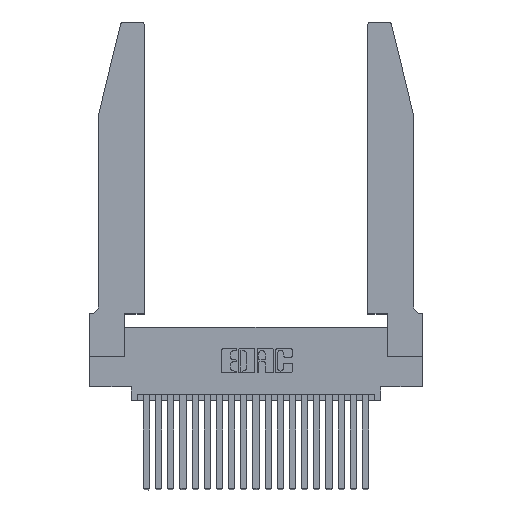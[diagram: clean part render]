
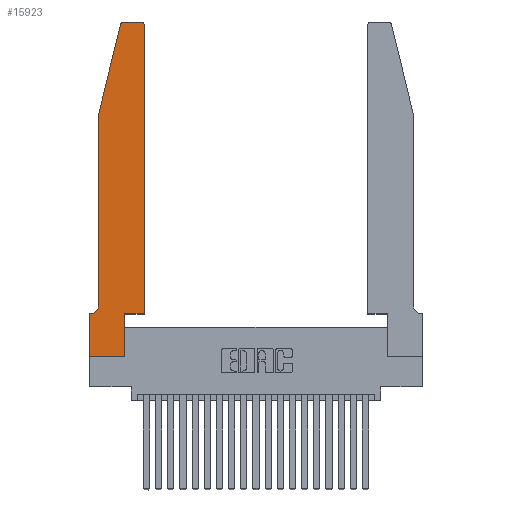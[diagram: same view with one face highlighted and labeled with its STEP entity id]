
A CAD part, top view. The second image highlights one B-rep face of the part: STEP entity #15923.
In plain terms, the highlighted planar face has unit normal (0, 0, 1).
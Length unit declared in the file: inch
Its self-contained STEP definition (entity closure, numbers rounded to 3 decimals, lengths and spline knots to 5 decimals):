
#23 = DIRECTION ( 'NONE',  ( 1., 0., 0. ) ) ;
#68 = EDGE_LOOP ( 'NONE', ( #13215, #6285, #16899, #22281, #315, #334, #8692, #9339, #8426, #6240, #14320, #22237 ) ) ;
#199 = DIRECTION ( 'NONE',  ( 1., 0., 0. ) ) ;
#242 = VECTOR ( 'NONE', #10638, 39.37008 ) ;
#315 = ORIENTED_EDGE ( 'NONE', *, *, #13425, .T. ) ;
#334 = ORIENTED_EDGE ( 'NONE', *, *, #4951, .T. ) ;
#385 = VERTEX_POINT ( 'NONE', #7137 ) ;
#736 = CARTESIAN_POINT ( 'NONE',  ( 0.4505, 0.35, 0.37 ) ) ;
#1230 = VECTOR ( 'NONE', #23, 39.37008 ) ;
#1583 = CARTESIAN_POINT ( 'NONE',  ( 0.4505, 0.35, 0.37 ) ) ;
#1658 = DIRECTION ( 'NONE',  ( 0., 0., 1. ) ) ;
#1879 = VERTEX_POINT ( 'NONE', #16109 ) ;
#2023 = CARTESIAN_POINT ( 'NONE',  ( 0., 0., 0.37 ) ) ;
#2698 = CARTESIAN_POINT ( 'NONE',  ( 0.0755, 2., 0.37 ) ) ;
#2812 = CARTESIAN_POINT ( 'NONE',  ( 0.284, 2.75, 0.37 ) ) ;
#2845 = EDGE_CURVE ( 'NONE', #11661, #4083, #5709, .T. ) ;
#2954 = PLANE ( 'NONE',  #10934 ) ;
#3644 = VECTOR ( 'NONE', #199, 39.37008 ) ;
#3740 = CARTESIAN_POINT ( 'NONE',  ( 0., 0., 0.37 ) ) ;
#3824 = CARTESIAN_POINT ( 'NONE',  ( 0.0755, 2., 0.37 ) ) ;
#4083 = VERTEX_POINT ( 'NONE', #2812 ) ;
#4455 = LINE ( 'NONE', #3824, #17082 ) ;
#4795 = VERTEX_POINT ( 'NONE', #22467 ) ;
#4796 = AXIS2_PLACEMENT_3D ( 'NONE', #5248, #1658, #10400 ) ;
#4951 = EDGE_CURVE ( 'NONE', #19156, #15522, #16598, .T. ) ;
#5170 = CARTESIAN_POINT ( 'NONE',  ( 0.0055, 0.35, 0.37 ) ) ;
#5248 = CARTESIAN_POINT ( 'NONE',  ( 0.284, 2.72, 0.37 ) ) ;
#5652 = EDGE_CURVE ( 'NONE', #4795, #11661, #22323, .T. ) ;
#5709 = LINE ( 'NONE', #21184, #242 ) ;
#5722 = CARTESIAN_POINT ( 'NONE',  ( 0.4505, 0.35, 0.37 ) ) ;
#6138 = DIRECTION ( 'NONE',  ( 1., 0., 0. ) ) ;
#6240 = ORIENTED_EDGE ( 'NONE', *, *, #19174, .T. ) ;
#6285 = ORIENTED_EDGE ( 'NONE', *, *, #20259, .T. ) ;
#6374 = EDGE_CURVE ( 'NONE', #9184, #7392, #6906, .T. ) ;
#6789 = DIRECTION ( 'NONE',  ( -1., 0., 0. ) ) ;
#6906 = LINE ( 'NONE', #3740, #3644 ) ;
#7137 = CARTESIAN_POINT ( 'NONE',  ( 0.25487, 2.72718, 0.37 ) ) ;
#7377 = CARTESIAN_POINT ( 'NONE',  ( 0.2865, 0., 0.37 ) ) ;
#7392 = VERTEX_POINT ( 'NONE', #7377 ) ;
#8208 = CARTESIAN_POINT ( 'NONE',  ( 0., 0.35, 0.37 ) ) ;
#8245 = LINE ( 'NONE', #14918, #15685 ) ;
#8426 = ORIENTED_EDGE ( 'NONE', *, *, #13246, .T. ) ;
#8542 = VERTEX_POINT ( 'NONE', #9794 ) ;
#8692 = ORIENTED_EDGE ( 'NONE', *, *, #11339, .T. ) ;
#9184 = VERTEX_POINT ( 'NONE', #2023 ) ;
#9339 = ORIENTED_EDGE ( 'NONE', *, *, #6374, .T. ) ;
#9432 = EDGE_CURVE ( 'NONE', #19937, #4795, #21313, .T. ) ;
#9520 = DIRECTION ( 'NONE',  ( 0., -1., 0. ) ) ;
#9662 = CIRCLE ( 'NONE', #12365, 0.07 ) ;
#9794 = CARTESIAN_POINT ( 'NONE',  ( 0.0755, 0.42, 0.37 ) ) ;
#10164 = DIRECTION ( 'NONE',  ( 0., 0., 1. ) ) ;
#10400 = DIRECTION ( 'NONE',  ( 1., 0., 0. ) ) ;
#10491 = CARTESIAN_POINT ( 'NONE',  ( 0.4205, 2.75, 0.37 ) ) ;
#10638 = DIRECTION ( 'NONE',  ( -1., 0., 0. ) ) ;
#10934 = AXIS2_PLACEMENT_3D ( 'NONE', #13537, #10164, #22427 ) ;
#11192 = CARTESIAN_POINT ( 'NONE',  ( 0.0055, 0.42, 0.37 ) ) ;
#11339 = EDGE_CURVE ( 'NONE', #15522, #9184, #11368, .T. ) ;
#11368 = LINE ( 'NONE', #14707, #22587 ) ;
#11377 = CARTESIAN_POINT ( 'NONE',  ( 0.4205, 2.72, 0.37 ) ) ;
#11661 = VERTEX_POINT ( 'NONE', #10491 ) ;
#11681 = DIRECTION ( 'NONE',  ( 0., -1., 0. ) ) ;
#11734 = VECTOR ( 'NONE', #11681, 39.37008 ) ;
#11840 = EDGE_CURVE ( 'NONE', #385, #15113, #4455, .T. ) ;
#11990 = VECTOR ( 'NONE', #14680, 39.37008 ) ;
#12365 = AXIS2_PLACEMENT_3D ( 'NONE', #11192, #14843, #21897 ) ;
#12826 = LINE ( 'NONE', #2698, #11734 ) ;
#13215 = ORIENTED_EDGE ( 'NONE', *, *, #2845, .T. ) ;
#13246 = EDGE_CURVE ( 'NONE', #7392, #1879, #8245, .T. ) ;
#13425 = EDGE_CURVE ( 'NONE', #8542, #19156, #9662, .T. ) ;
#13537 = CARTESIAN_POINT ( 'NONE',  ( 0., 0.35, 0.37 ) ) ;
#14320 = ORIENTED_EDGE ( 'NONE', *, *, #9432, .T. ) ;
#14680 = DIRECTION ( 'NONE',  ( 0., 1., 0. ) ) ;
#14707 = CARTESIAN_POINT ( 'NONE',  ( 0., 0., 0.37 ) ) ;
#14843 = DIRECTION ( 'NONE',  ( 0., 0., -1. ) ) ;
#14870 = DIRECTION ( 'NONE',  ( 0., 0., 1. ) ) ;
#14918 = CARTESIAN_POINT ( 'NONE',  ( 0.2865, 0.35, 0.37 ) ) ;
#15113 = VERTEX_POINT ( 'NONE', #21709 ) ;
#15132 = AXIS2_PLACEMENT_3D ( 'NONE', #11377, #14870, #6138 ) ;
#15522 = VERTEX_POINT ( 'NONE', #8208 ) ;
#15685 = VECTOR ( 'NONE', #20204, 39.37008 ) ;
#15923 = ADVANCED_FACE ( 'NONE', ( #18914 ), #2954, .T. ) ;
#16109 = CARTESIAN_POINT ( 'NONE',  ( 0.2865, 0.35, 0.37 ) ) ;
#16598 = LINE ( 'NONE', #17532, #22370 ) ;
#16899 = ORIENTED_EDGE ( 'NONE', *, *, #11840, .T. ) ;
#17082 = VECTOR ( 'NONE', #17824, 39.37008 ) ;
#17532 = CARTESIAN_POINT ( 'NONE',  ( 0.0755, 0.35, 0.37 ) ) ;
#17824 = DIRECTION ( 'NONE',  ( -0.239, -0.971, 0. ) ) ;
#17965 = EDGE_CURVE ( 'NONE', #15113, #8542, #12826, .T. ) ;
#18730 = CIRCLE ( 'NONE', #4796, 0.03 ) ;
#18914 = FACE_OUTER_BOUND ( 'NONE', #68, .T. ) ;
#19156 = VERTEX_POINT ( 'NONE', #5170 ) ;
#19174 = EDGE_CURVE ( 'NONE', #1879, #19937, #21534, .T. ) ;
#19937 = VERTEX_POINT ( 'NONE', #736 ) ;
#20204 = DIRECTION ( 'NONE',  ( 0., 1., 0. ) ) ;
#20259 = EDGE_CURVE ( 'NONE', #4083, #385, #18730, .T. ) ;
#21184 = CARTESIAN_POINT ( 'NONE',  ( 0.2605, 2.75, 0.37 ) ) ;
#21313 = LINE ( 'NONE', #5722, #11990 ) ;
#21534 = LINE ( 'NONE', #1583, #1230 ) ;
#21709 = CARTESIAN_POINT ( 'NONE',  ( 0.0755, 2., 0.37 ) ) ;
#21897 = DIRECTION ( 'NONE',  ( -1., 0., 0. ) ) ;
#22237 = ORIENTED_EDGE ( 'NONE', *, *, #5652, .T. ) ;
#22281 = ORIENTED_EDGE ( 'NONE', *, *, #17965, .T. ) ;
#22323 = CIRCLE ( 'NONE', #15132, 0.03 ) ;
#22370 = VECTOR ( 'NONE', #6789, 39.37008 ) ;
#22427 = DIRECTION ( 'NONE',  ( 1., 0., 0. ) ) ;
#22467 = CARTESIAN_POINT ( 'NONE',  ( 0.4505, 2.72, 0.37 ) ) ;
#22587 = VECTOR ( 'NONE', #9520, 39.37008 ) ;
